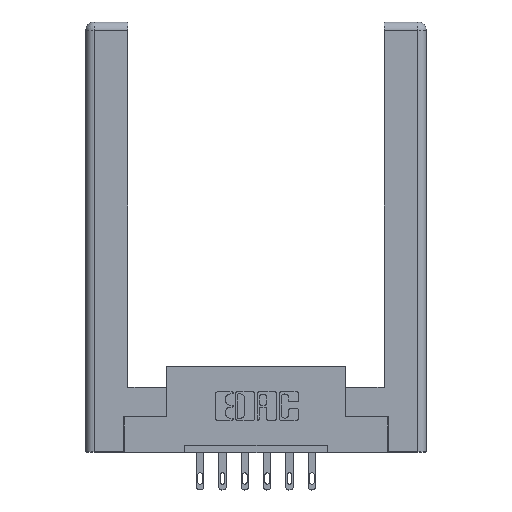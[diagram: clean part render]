
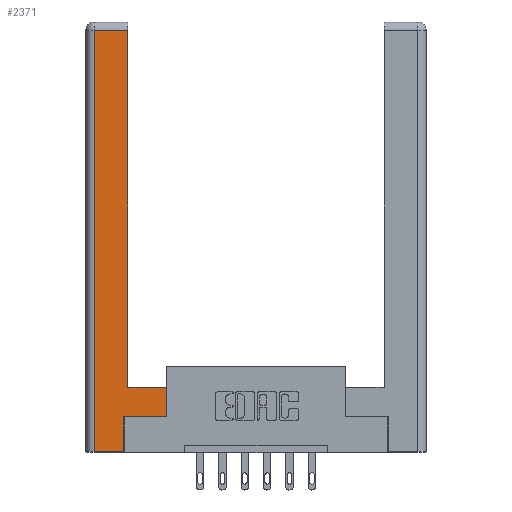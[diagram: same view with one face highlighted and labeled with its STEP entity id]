
A CAD part, top view. The second image highlights one B-rep face of the part: STEP entity #2371.
In plain terms, the highlighted planar face has unit normal (0, 0, 1).
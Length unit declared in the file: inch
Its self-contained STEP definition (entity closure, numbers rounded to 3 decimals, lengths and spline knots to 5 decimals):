
#467 = CARTESIAN_POINT ( 'NONE',  ( 0.565, 0.245, 0. ) ) ;
#515 = ORIENTED_EDGE ( 'NONE', *, *, #3801, .T. ) ;
#589 = EDGE_CURVE ( 'NONE', #5148, #4671, #3921, .T. ) ;
#632 = ORIENTED_EDGE ( 'NONE', *, *, #1483, .T. ) ;
#954 = DIRECTION ( 'NONE',  ( 0., -1., 0. ) ) ;
#1379 = VECTOR ( 'NONE', #2197, 39.37008 ) ;
#1394 = CARTESIAN_POINT ( 'NONE',  ( 0.295, 2.94, 0. ) ) ;
#1468 = EDGE_CURVE ( 'NONE', #1947, #3555, #9563, .T. ) ;
#1483 = EDGE_CURVE ( 'NONE', #5855, #9750, #7140, .T. ) ;
#1572 = ORIENTED_EDGE ( 'NONE', *, *, #10146, .T. ) ;
#1606 = DIRECTION ( 'NONE',  ( 0., 1., 0. ) ) ;
#1652 = LINE ( 'NONE', #6760, #1379 ) ;
#1947 = VERTEX_POINT ( 'NONE', #1394 ) ;
#2197 = DIRECTION ( 'NONE',  ( 1., 0., 0. ) ) ;
#2199 = CARTESIAN_POINT ( 'NONE',  ( 0.295, 0.45, 0. ) ) ;
#2366 = VECTOR ( 'NONE', #3320, 39.37008 ) ;
#2371 = ADVANCED_FACE ( 'NONE', ( #10392 ), #4830, .F. ) ;
#2963 = ORIENTED_EDGE ( 'NONE', *, *, #8968, .T. ) ;
#3006 = LINE ( 'NONE', #4841, #3869 ) ;
#3216 = VECTOR ( 'NONE', #10545, 39.37008 ) ;
#3320 = DIRECTION ( 'NONE',  ( 0., 1., 0. ) ) ;
#3434 = CARTESIAN_POINT ( 'NONE',  ( 0.565, 0.45, 0. ) ) ;
#3525 = CARTESIAN_POINT ( 'NONE',  ( 0.265, 0.245, 0. ) ) ;
#3526 = CARTESIAN_POINT ( 'NONE',  ( 0.565, 0.45, 0. ) ) ;
#3555 = VERTEX_POINT ( 'NONE', #6782 ) ;
#3801 = EDGE_CURVE ( 'NONE', #11159, #1947, #10207, .T. ) ;
#3869 = VECTOR ( 'NONE', #10147, 39.37008 ) ;
#3921 = LINE ( 'NONE', #3525, #7736 ) ;
#4125 = VECTOR ( 'NONE', #4176, 39.37008 ) ;
#4176 = DIRECTION ( 'NONE',  ( 0., 1., 0. ) ) ;
#4338 = ORIENTED_EDGE ( 'NONE', *, *, #5445, .T. ) ;
#4442 = CARTESIAN_POINT ( 'NONE',  ( 0.0615, 0., 0. ) ) ;
#4671 = VERTEX_POINT ( 'NONE', #6064 ) ;
#4830 = PLANE ( 'NONE',  #6849 ) ;
#4841 = CARTESIAN_POINT ( 'NONE',  ( 0.295, 0.45, 0. ) ) ;
#4950 = DIRECTION ( 'NONE',  ( -1., 0., 0. ) ) ;
#5148 = VERTEX_POINT ( 'NONE', #5977 ) ;
#5445 = EDGE_CURVE ( 'NONE', #3555, #10929, #5812, .T. ) ;
#5600 = LINE ( 'NONE', #7898, #3216 ) ;
#5812 = LINE ( 'NONE', #10801, #7228 ) ;
#5855 = VERTEX_POINT ( 'NONE', #467 ) ;
#5977 = CARTESIAN_POINT ( 'NONE',  ( 0.265, 0., 0. ) ) ;
#6064 = CARTESIAN_POINT ( 'NONE',  ( 0.265, 0.245, 0. ) ) ;
#6145 = CARTESIAN_POINT ( 'NONE',  ( 0.295, 3., 0. ) ) ;
#6760 = CARTESIAN_POINT ( 'NONE',  ( 0.265, 0., 0. ) ) ;
#6782 = CARTESIAN_POINT ( 'NONE',  ( 0.0615, 2.94, 0. ) ) ;
#6849 = AXIS2_PLACEMENT_3D ( 'NONE', #9462, #10378, #4950 ) ;
#7140 = LINE ( 'NONE', #3434, #2366 ) ;
#7228 = VECTOR ( 'NONE', #954, 39.37008 ) ;
#7416 = ORIENTED_EDGE ( 'NONE', *, *, #589, .T. ) ;
#7483 = EDGE_LOOP ( 'NONE', ( #515, #9890, #4338, #2963, #7416, #9304, #632, #1572 ) ) ;
#7736 = VECTOR ( 'NONE', #1606, 39.37008 ) ;
#7898 = CARTESIAN_POINT ( 'NONE',  ( 0.565, 0.245, 0. ) ) ;
#7909 = EDGE_CURVE ( 'NONE', #4671, #5855, #5600, .T. ) ;
#8106 = DIRECTION ( 'NONE',  ( -1., 0., 0. ) ) ;
#8221 = CARTESIAN_POINT ( 'NONE',  ( 0.0615, 2.94, 0. ) ) ;
#8968 = EDGE_CURVE ( 'NONE', #10929, #5148, #1652, .T. ) ;
#9304 = ORIENTED_EDGE ( 'NONE', *, *, #7909, .T. ) ;
#9462 = CARTESIAN_POINT ( 'NONE',  ( 0., 0., 0. ) ) ;
#9563 = LINE ( 'NONE', #8221, #10688 ) ;
#9750 = VERTEX_POINT ( 'NONE', #3526 ) ;
#9890 = ORIENTED_EDGE ( 'NONE', *, *, #1468, .T. ) ;
#10146 = EDGE_CURVE ( 'NONE', #9750, #11159, #3006, .T. ) ;
#10147 = DIRECTION ( 'NONE',  ( -1., 0., 0. ) ) ;
#10207 = LINE ( 'NONE', #6145, #4125 ) ;
#10378 = DIRECTION ( 'NONE',  ( 0., 0., -1. ) ) ;
#10392 = FACE_OUTER_BOUND ( 'NONE', #7483, .T. ) ;
#10545 = DIRECTION ( 'NONE',  ( 1., 0., 0. ) ) ;
#10688 = VECTOR ( 'NONE', #8106, 39.37008 ) ;
#10801 = CARTESIAN_POINT ( 'NONE',  ( 0.0615, 0., 0. ) ) ;
#10929 = VERTEX_POINT ( 'NONE', #4442 ) ;
#11159 = VERTEX_POINT ( 'NONE', #2199 ) ;
